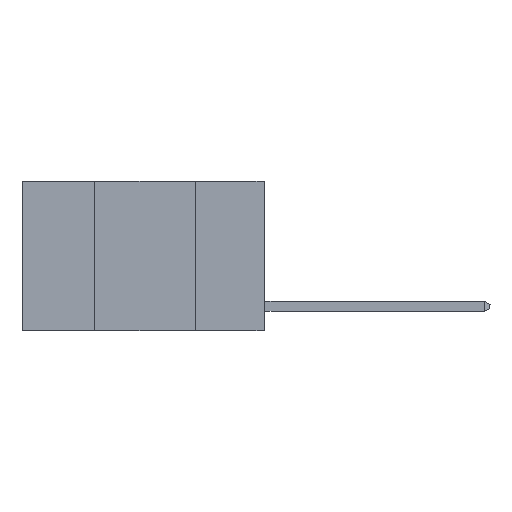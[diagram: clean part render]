
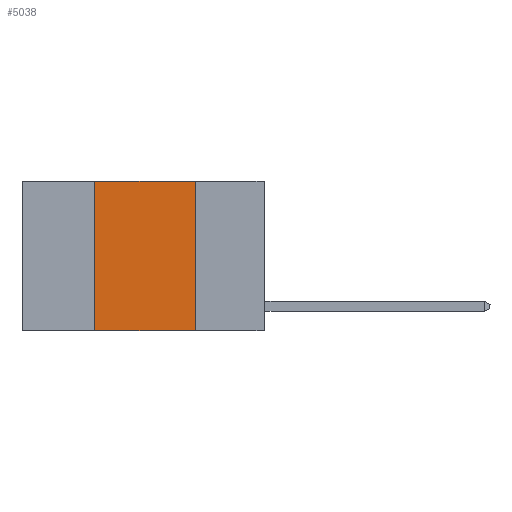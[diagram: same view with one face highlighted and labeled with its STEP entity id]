
A CAD part, left-side view. The second image highlights one B-rep face of the part: STEP entity #5038.
In plain terms, the highlighted planar face has unit normal (-1, 0, 0).
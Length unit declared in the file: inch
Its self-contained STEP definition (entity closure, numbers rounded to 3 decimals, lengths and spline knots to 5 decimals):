
#19 = VERTEX_POINT ( 'NONE', #2734 ) ;
#57 = DIRECTION ( 'NONE',  ( 0., -1., 0. ) ) ;
#552 = CARTESIAN_POINT ( 'NONE',  ( 0., 0.42, 0. ) ) ;
#1793 = DIRECTION ( 'NONE',  ( 0., -1., 0. ) ) ;
#2479 = DIRECTION ( 'NONE',  ( 0., 0., 1. ) ) ;
#2734 = CARTESIAN_POINT ( 'NONE',  ( 0., 0.42, -0.37 ) ) ;
#2811 = CARTESIAN_POINT ( 'NONE',  ( 0., 0.6, -0.37 ) ) ;
#3321 = FACE_OUTER_BOUND ( 'NONE', #16624, .T. ) ;
#3415 = VECTOR ( 'NONE', #2479, 39.37008 ) ;
#3426 = VECTOR ( 'NONE', #57, 39.37008 ) ;
#4411 = EDGE_CURVE ( 'NONE', #10290, #4696, #16094, .T. ) ;
#4696 = VERTEX_POINT ( 'NONE', #16556 ) ;
#5038 = ADVANCED_FACE ( 'NONE', ( #3321 ), #11005, .F. ) ;
#5155 = ORIENTED_EDGE ( 'NONE', *, *, #13277, .T. ) ;
#5587 = EDGE_CURVE ( 'NONE', #4696, #16723, #9244, .T. ) ;
#6380 = CARTESIAN_POINT ( 'NONE',  ( 0., 0.17, 0. ) ) ;
#6476 = VECTOR ( 'NONE', #1793, 39.37008 ) ;
#7370 = CARTESIAN_POINT ( 'NONE',  ( 0., 0.6, 0. ) ) ;
#8489 = LINE ( 'NONE', #2811, #3426 ) ;
#8538 = LINE ( 'NONE', #15621, #3415 ) ;
#9171 = CARTESIAN_POINT ( 'NONE',  ( 0., 0.6, 0. ) ) ;
#9244 = LINE ( 'NONE', #6380, #15787 ) ;
#9456 = DIRECTION ( 'NONE',  ( 0., 0., -1. ) ) ;
#10290 = VERTEX_POINT ( 'NONE', #552 ) ;
#10998 = CARTESIAN_POINT ( 'NONE',  ( 0., 0.17, -0.37 ) ) ;
#11005 = PLANE ( 'NONE',  #14810 ) ;
#12429 = DIRECTION ( 'NONE',  ( 1., 0., 0. ) ) ;
#13277 = EDGE_CURVE ( 'NONE', #19, #16723, #8489, .T. ) ;
#13619 = ORIENTED_EDGE ( 'NONE', *, *, #5587, .F. ) ;
#14147 = EDGE_CURVE ( 'NONE', #19, #10290, #8538, .T. ) ;
#14810 = AXIS2_PLACEMENT_3D ( 'NONE', #9171, #12429, #9456 ) ;
#14951 = ORIENTED_EDGE ( 'NONE', *, *, #4411, .F. ) ;
#15057 = DIRECTION ( 'NONE',  ( 0., 0., -1. ) ) ;
#15621 = CARTESIAN_POINT ( 'NONE',  ( 0., 0.42, 0. ) ) ;
#15787 = VECTOR ( 'NONE', #15057, 39.37008 ) ;
#16094 = LINE ( 'NONE', #7370, #6476 ) ;
#16556 = CARTESIAN_POINT ( 'NONE',  ( 0., 0.17, 0. ) ) ;
#16624 = EDGE_LOOP ( 'NONE', ( #13619, #14951, #17729, #5155 ) ) ;
#16723 = VERTEX_POINT ( 'NONE', #10998 ) ;
#17729 = ORIENTED_EDGE ( 'NONE', *, *, #14147, .F. ) ;
